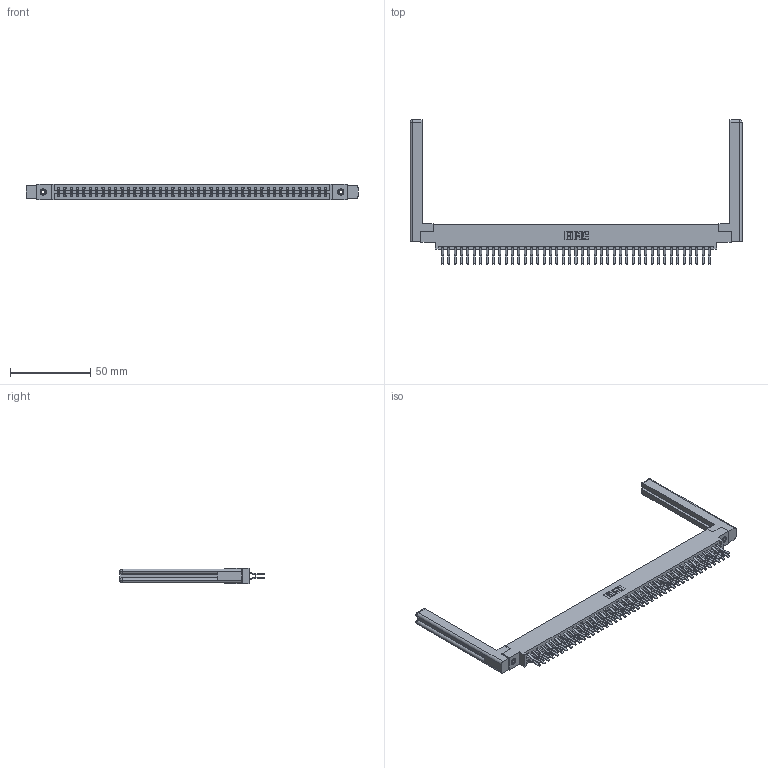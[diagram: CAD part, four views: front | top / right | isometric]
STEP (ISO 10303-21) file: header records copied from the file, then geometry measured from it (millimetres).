
FILE_DESCRIPTION (( 'STEP AP203' ), '1' );
FILE_NAME ('387-086-560-858.STEP', '2019-10-23T04:54:12', ( '' ), ( '' ), 'SwSTEP 2.0', 'SolidWorks 2016', '' );
FILE_SCHEMA (( 'CONFIG_CONTROL_DESIGN' ));
Length unit declared in the file: inch
Products named in the file (5): 307-220-058; 345-250-001_345-250-001-102; 387-086-560-858; 345-292-001_560 Tail; 337 Part_0.170 Offset - 0.156 Dia-TI
Assembly tree (91 placements, depth 2):
  387-086-560-858
    337 Part_0.170 Offset - 0.156 Dia-TI
    345-292-001_560 Tail  x86
    345-250-001_345-250-001-102  x2
    307-220-058  x2
Bounding box: 207.01 x 90.19 x 9.4 mm (x, y, z)
Volume: 29418.2 mm3; surface area: 31978.7 mm2
Topology: 91 solids, 91 shells, 5076 faces, 15039 edges, 9898 vertices
Faces by surface type: plane 3426, cylinder 1626, cone 12, torus 12
Entity records: 36064 total; most frequent: CARTESIAN_POINT 6085, ORIENTED_EDGE 5960, DIRECTION 5192, EDGE_CURVE 2980, VECTOR 2800, LINE 2800, VERTEX_POINT 1978, AXIS2_PLACEMENT_3D 1196
